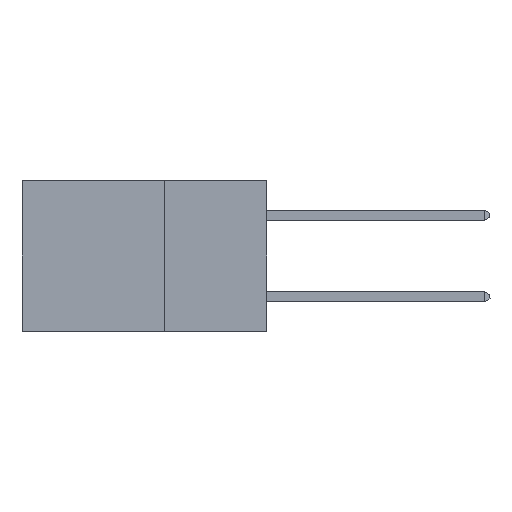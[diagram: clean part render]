
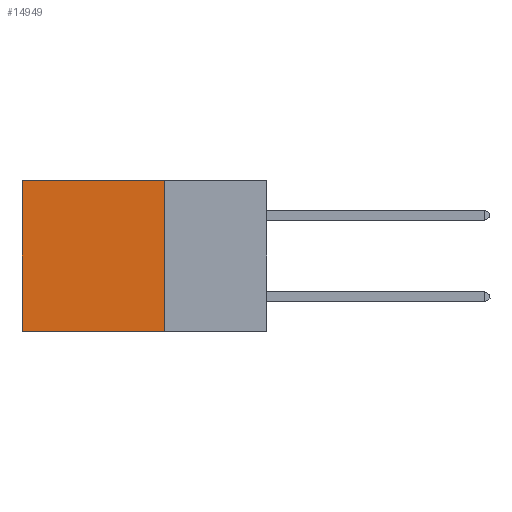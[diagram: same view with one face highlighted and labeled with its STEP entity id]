
A CAD part, left-side view. The second image highlights one B-rep face of the part: STEP entity #14949.
In plain terms, the highlighted planar face has unit normal (-1, 0, 0).
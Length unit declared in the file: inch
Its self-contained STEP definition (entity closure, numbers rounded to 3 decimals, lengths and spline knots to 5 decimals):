
#1884 = LINE ( 'NONE', #17716, #9308 ) ;
#2026 = ORIENTED_EDGE ( 'NONE', *, *, #16458, .F. ) ;
#2774 = ORIENTED_EDGE ( 'NONE', *, *, #8169, .F. ) ;
#2992 = FACE_OUTER_BOUND ( 'NONE', #12778, .T. ) ;
#3610 = VERTEX_POINT ( 'NONE', #7063 ) ;
#4920 = EDGE_CURVE ( 'NONE', #15164, #14282, #8308, .T. ) ;
#4979 = DIRECTION ( 'NONE',  ( 0., 0., -1. ) ) ;
#5353 = CARTESIAN_POINT ( 'NONE',  ( 0.2875, 0.25, -0.37 ) ) ;
#6543 = PLANE ( 'NONE',  #9459 ) ;
#6967 = DIRECTION ( 'NONE',  ( 0., 1., 0. ) ) ;
#7063 = CARTESIAN_POINT ( 'NONE',  ( 0.2875, 0.25, -0.37 ) ) ;
#7134 = VECTOR ( 'NONE', #6967, 39.37008 ) ;
#7787 = VECTOR ( 'NONE', #10821, 39.37008 ) ;
#8155 = CARTESIAN_POINT ( 'NONE',  ( 0.2875, 0.25, 0. ) ) ;
#8169 = EDGE_CURVE ( 'NONE', #15164, #3610, #14878, .T. ) ;
#8308 = LINE ( 'NONE', #14006, #7787 ) ;
#9308 = VECTOR ( 'NONE', #19339, 39.37008 ) ;
#9410 = ORIENTED_EDGE ( 'NONE', *, *, #4920, .T. ) ;
#9459 = AXIS2_PLACEMENT_3D ( 'NONE', #8155, #19320, #9764 ) ;
#9584 = ORIENTED_EDGE ( 'NONE', *, *, #12062, .T. ) ;
#9764 = DIRECTION ( 'NONE',  ( 0., 0., -1. ) ) ;
#10586 = VECTOR ( 'NONE', #4979, 39.37008 ) ;
#10821 = DIRECTION ( 'NONE',  ( 0., 1., 0. ) ) ;
#11920 = CARTESIAN_POINT ( 'NONE',  ( 0.2875, 0.25, 0. ) ) ;
#12062 = EDGE_CURVE ( 'NONE', #14282, #16369, #1884, .T. ) ;
#12778 = EDGE_LOOP ( 'NONE', ( #9584, #2026, #2774, #9410 ) ) ;
#14006 = CARTESIAN_POINT ( 'NONE',  ( 0.2875, 0.25, 0. ) ) ;
#14083 = CARTESIAN_POINT ( 'NONE',  ( 0.2875, 0.6, 0. ) ) ;
#14282 = VERTEX_POINT ( 'NONE', #14083 ) ;
#14878 = LINE ( 'NONE', #17681, #10586 ) ;
#14949 = ADVANCED_FACE ( 'NONE', ( #2992 ), #6543, .F. ) ;
#15164 = VERTEX_POINT ( 'NONE', #11920 ) ;
#15668 = LINE ( 'NONE', #5353, #7134 ) ;
#16275 = CARTESIAN_POINT ( 'NONE',  ( 0.2875, 0.6, -0.37 ) ) ;
#16369 = VERTEX_POINT ( 'NONE', #16275 ) ;
#16458 = EDGE_CURVE ( 'NONE', #3610, #16369, #15668, .T. ) ;
#17681 = CARTESIAN_POINT ( 'NONE',  ( 0.2875, 0.25, 0. ) ) ;
#17716 = CARTESIAN_POINT ( 'NONE',  ( 0.2875, 0.6, 0. ) ) ;
#19320 = DIRECTION ( 'NONE',  ( 1., 0., 0. ) ) ;
#19339 = DIRECTION ( 'NONE',  ( 0., 0., -1. ) ) ;
